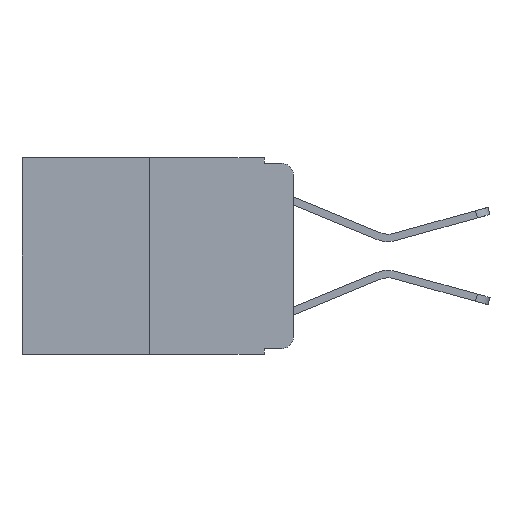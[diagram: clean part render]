
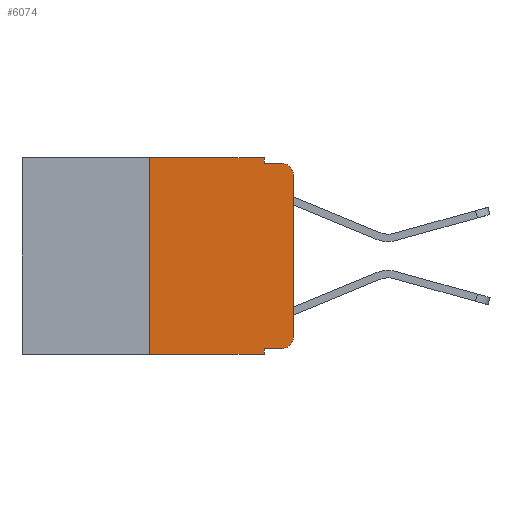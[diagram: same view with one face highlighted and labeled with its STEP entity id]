
A CAD part, left-side view. The second image highlights one B-rep face of the part: STEP entity #6074.
In plain terms, the highlighted planar face has unit normal (-1, 0, 0).
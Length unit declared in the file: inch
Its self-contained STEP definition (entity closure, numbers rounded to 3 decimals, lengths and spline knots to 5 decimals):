
#4 = VERTEX_POINT ( 'NONE', #3313 ) ;
#28 = ORIENTED_EDGE ( 'NONE', *, *, #12797, .T. ) ;
#140 = EDGE_CURVE ( 'NONE', #8109, #9875, #10703, .T. ) ;
#1710 = DIRECTION ( 'NONE',  ( 0., 0., -1. ) ) ;
#2348 = CIRCLE ( 'NONE', #14536, 0.02 ) ;
#2390 = VECTOR ( 'NONE', #17455, 39.37008 ) ;
#3313 = CARTESIAN_POINT ( 'NONE',  ( 0., 0., -0.03 ) ) ;
#4097 = CARTESIAN_POINT ( 'NONE',  ( 0., 0.473, 0. ) ) ;
#4634 = CARTESIAN_POINT ( 'NONE',  ( 0., 0.473, -0.343 ) ) ;
#4708 = CIRCLE ( 'NONE', #20625, 0.02 ) ;
#4712 = VECTOR ( 'NONE', #12787, 39.37008 ) ;
#4945 = AXIS2_PLACEMENT_3D ( 'NONE', #4097, #15488, #5870 ) ;
#5066 = CARTESIAN_POINT ( 'NONE',  ( 0., 0.25, 0. ) ) ;
#5269 = CARTESIAN_POINT ( 'NONE',  ( 0., 0.02, -0.333 ) ) ;
#5562 = CARTESIAN_POINT ( 'NONE',  ( 0., 0.051, -0.343 ) ) ;
#5618 = CARTESIAN_POINT ( 'NONE',  ( 0., 0.25, -0.343 ) ) ;
#5791 = ORIENTED_EDGE ( 'NONE', *, *, #20795, .T. ) ;
#5870 = DIRECTION ( 'NONE',  ( 0., 0., -1. ) ) ;
#6074 = ADVANCED_FACE ( 'NONE', ( #12409 ), #17263, .F. ) ;
#6112 = CARTESIAN_POINT ( 'NONE',  ( 0., 0.051, -0.333 ) ) ;
#6586 = VECTOR ( 'NONE', #7554, 39.37008 ) ;
#6615 = ORIENTED_EDGE ( 'NONE', *, *, #18535, .F. ) ;
#7554 = DIRECTION ( 'NONE',  ( 0., 0., -1. ) ) ;
#7813 = DIRECTION ( 'NONE',  ( -1., 0., 0. ) ) ;
#8109 = VERTEX_POINT ( 'NONE', #5618 ) ;
#8168 = DIRECTION ( 'NONE',  ( -1., 0., 0. ) ) ;
#8333 = ORIENTED_EDGE ( 'NONE', *, *, #19082, .T. ) ;
#8914 = DIRECTION ( 'NONE',  ( 0., 0., 1. ) ) ;
#9029 = LINE ( 'NONE', #11157, #4712 ) ;
#9166 = CARTESIAN_POINT ( 'NONE',  ( 0., 0.473, 0. ) ) ;
#9334 = VECTOR ( 'NONE', #19130, 39.37008 ) ;
#9597 = VERTEX_POINT ( 'NONE', #5066 ) ;
#9875 = VERTEX_POINT ( 'NONE', #5562 ) ;
#10083 = DIRECTION ( 'NONE',  ( 0., -1., 0. ) ) ;
#10467 = CARTESIAN_POINT ( 'NONE',  ( 0., 0.25, 0. ) ) ;
#10685 = ORIENTED_EDGE ( 'NONE', *, *, #140, .T. ) ;
#10703 = LINE ( 'NONE', #4634, #14528 ) ;
#10863 = LINE ( 'NONE', #10467, #12647 ) ;
#11054 = DIRECTION ( 'NONE',  ( 0., 0., -1. ) ) ;
#11157 = CARTESIAN_POINT ( 'NONE',  ( 0., 0., 0. ) ) ;
#11202 = CARTESIAN_POINT ( 'NONE',  ( 0., 0.051, -0.01 ) ) ;
#11287 = ORIENTED_EDGE ( 'NONE', *, *, #11483, .F. ) ;
#11305 = CARTESIAN_POINT ( 'NONE',  ( 0., 0.051, -0.01 ) ) ;
#11483 = EDGE_CURVE ( 'NONE', #18276, #9875, #13200, .T. ) ;
#11729 = VERTEX_POINT ( 'NONE', #19529 ) ;
#11777 = ORIENTED_EDGE ( 'NONE', *, *, #15231, .F. ) ;
#11779 = ORIENTED_EDGE ( 'NONE', *, *, #15759, .F. ) ;
#12089 = LINE ( 'NONE', #11305, #18463 ) ;
#12409 = FACE_OUTER_BOUND ( 'NONE', #16553, .T. ) ;
#12647 = VECTOR ( 'NONE', #8914, 39.37008 ) ;
#12705 = EDGE_CURVE ( 'NONE', #8109, #9597, #10863, .T. ) ;
#12787 = DIRECTION ( 'NONE',  ( 0., 0., 1. ) ) ;
#12797 = EDGE_CURVE ( 'NONE', #18276, #18056, #16742, .T. ) ;
#13037 = ORIENTED_EDGE ( 'NONE', *, *, #14118, .T. ) ;
#13200 = LINE ( 'NONE', #18841, #6586 ) ;
#13317 = CARTESIAN_POINT ( 'NONE',  ( 0., 0.02, -0.01 ) ) ;
#13530 = LINE ( 'NONE', #9166, #16085 ) ;
#13730 = DIRECTION ( 'NONE',  ( 0., -1., 0. ) ) ;
#14118 = EDGE_CURVE ( 'NONE', #11729, #4, #9029, .T. ) ;
#14436 = CARTESIAN_POINT ( 'NONE',  ( 0., 0.051, 0. ) ) ;
#14528 = VECTOR ( 'NONE', #20890, 39.37008 ) ;
#14536 = AXIS2_PLACEMENT_3D ( 'NONE', #15892, #7813, #11054 ) ;
#14699 = VERTEX_POINT ( 'NONE', #11202 ) ;
#14811 = LINE ( 'NONE', #15807, #2390 ) ;
#15231 = EDGE_CURVE ( 'NONE', #19674, #14699, #14811, .T. ) ;
#15488 = DIRECTION ( 'NONE',  ( 1., 0., 0. ) ) ;
#15759 = EDGE_CURVE ( 'NONE', #9597, #19674, #13530, .T. ) ;
#15807 = CARTESIAN_POINT ( 'NONE',  ( 0., 0.051, 0. ) ) ;
#15892 = CARTESIAN_POINT ( 'NONE',  ( 0., 0.02, -0.03 ) ) ;
#16085 = VECTOR ( 'NONE', #13730, 39.37008 ) ;
#16553 = EDGE_LOOP ( 'NONE', ( #13037, #5791, #6615, #11777, #11779, #20103, #10685, #11287, #28, #8333 ) ) ;
#16742 = LINE ( 'NONE', #18922, #9334 ) ;
#17263 = PLANE ( 'NONE',  #4945 ) ;
#17455 = DIRECTION ( 'NONE',  ( 0., 0., -1. ) ) ;
#18056 = VERTEX_POINT ( 'NONE', #5269 ) ;
#18276 = VERTEX_POINT ( 'NONE', #6112 ) ;
#18463 = VECTOR ( 'NONE', #10083, 39.37008 ) ;
#18535 = EDGE_CURVE ( 'NONE', #14699, #19321, #12089, .T. ) ;
#18841 = CARTESIAN_POINT ( 'NONE',  ( 0., 0.051, 0. ) ) ;
#18922 = CARTESIAN_POINT ( 'NONE',  ( 0., 0.051, -0.333 ) ) ;
#19082 = EDGE_CURVE ( 'NONE', #18056, #11729, #4708, .T. ) ;
#19130 = DIRECTION ( 'NONE',  ( 0., -1., 0. ) ) ;
#19321 = VERTEX_POINT ( 'NONE', #13317 ) ;
#19529 = CARTESIAN_POINT ( 'NONE',  ( 0., 0., -0.313 ) ) ;
#19674 = VERTEX_POINT ( 'NONE', #14436 ) ;
#19802 = CARTESIAN_POINT ( 'NONE',  ( 0., 0.02, -0.313 ) ) ;
#20103 = ORIENTED_EDGE ( 'NONE', *, *, #12705, .F. ) ;
#20625 = AXIS2_PLACEMENT_3D ( 'NONE', #19802, #8168, #1710 ) ;
#20795 = EDGE_CURVE ( 'NONE', #4, #19321, #2348, .T. ) ;
#20890 = DIRECTION ( 'NONE',  ( 0., -1., 0. ) ) ;
